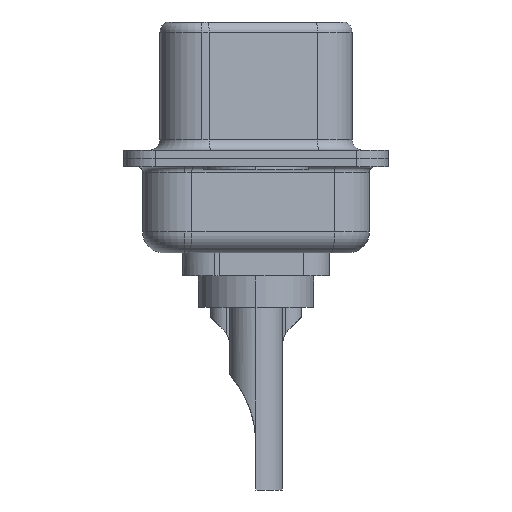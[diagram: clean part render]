
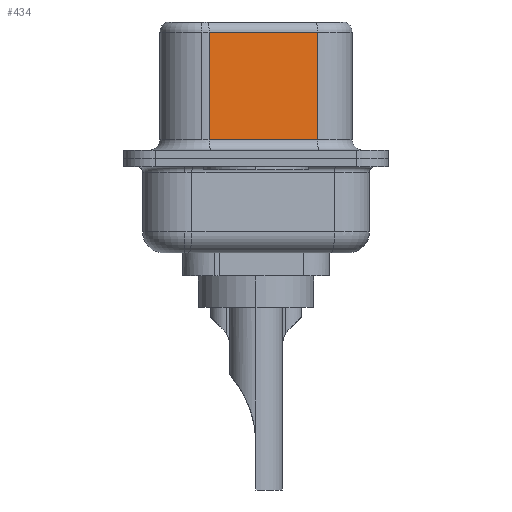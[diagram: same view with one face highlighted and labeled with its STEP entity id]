
A CAD part, left-side view. The second image highlights one B-rep face of the part: STEP entity #434.
In plain terms, the highlighted planar face has unit normal (-0.985, -0.174, 0).
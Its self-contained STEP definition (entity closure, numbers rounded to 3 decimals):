
#17 = DIRECTION ( 'NONE',  ( -0.174, 0.985, 0. ) ) ;
#160 = CARTESIAN_POINT ( 'NONE',  ( 4.565, -2.927, 0.9 ) ) ;
#434 = ADVANCED_FACE ( 'NONE', ( #3321 ), #920, .F. ) ;
#579 = EDGE_CURVE ( 'NONE', #1395, #7417, #12391, .T. ) ;
#673 = LINE ( 'NONE', #160, #12047 ) ;
#817 = DIRECTION ( 'NONE',  ( 0.985, 0.174, 0. ) ) ;
#920 = PLANE ( 'NONE',  #6382 ) ;
#986 = CARTESIAN_POINT ( 'NONE',  ( 4.565, -2.927, 6.02 ) ) ;
#1395 = VERTEX_POINT ( 'NONE', #13186 ) ;
#1412 = CARTESIAN_POINT ( 'NONE',  ( 4.565, -2.927, 6.52 ) ) ;
#2065 = EDGE_CURVE ( 'NONE', #7417, #7648, #2249, .T. ) ;
#2125 = DIRECTION ( 'NONE',  ( -0.174, 0.985, 0. ) ) ;
#2249 = LINE ( 'NONE', #8790, #13193 ) ;
#2367 = DIRECTION ( 'NONE',  ( 0., 0., -1. ) ) ;
#3171 = ORIENTED_EDGE ( 'NONE', *, *, #2065, .T. ) ;
#3321 = FACE_OUTER_BOUND ( 'NONE', #6710, .T. ) ;
#3608 = DIRECTION ( 'NONE',  ( 0., 0., -1. ) ) ;
#3700 = VECTOR ( 'NONE', #2367, 1000. ) ;
#5570 = ORIENTED_EDGE ( 'NONE', *, *, #9872, .F. ) ;
#5875 = CARTESIAN_POINT ( 'NONE',  ( 3.655, 2.233, 6.02 ) ) ;
#6197 = CARTESIAN_POINT ( 'NONE',  ( 3.655, 2.233, 0.9 ) ) ;
#6382 = AXIS2_PLACEMENT_3D ( 'NONE', #1412, #817, #2125 ) ;
#6707 = LINE ( 'NONE', #12182, #3700 ) ;
#6710 = EDGE_LOOP ( 'NONE', ( #5570, #9711, #3171, #8207 ) ) ;
#7417 = VERTEX_POINT ( 'NONE', #5875 ) ;
#7648 = VERTEX_POINT ( 'NONE', #6197 ) ;
#7986 = DIRECTION ( 'NONE',  ( 0.174, -0.985, 0. ) ) ;
#8207 = ORIENTED_EDGE ( 'NONE', *, *, #9887, .T. ) ;
#8790 = CARTESIAN_POINT ( 'NONE',  ( 3.655, 2.233, 6.52 ) ) ;
#9711 = ORIENTED_EDGE ( 'NONE', *, *, #579, .T. ) ;
#9847 = VECTOR ( 'NONE', #17, 1000. ) ;
#9872 = EDGE_CURVE ( 'NONE', #1395, #13435, #6707, .T. ) ;
#9887 = EDGE_CURVE ( 'NONE', #7648, #13435, #673, .T. ) ;
#12047 = VECTOR ( 'NONE', #7986, 1000. ) ;
#12182 = CARTESIAN_POINT ( 'NONE',  ( 4.565, -2.927, 6.52 ) ) ;
#12391 = LINE ( 'NONE', #986, #9847 ) ;
#12587 = CARTESIAN_POINT ( 'NONE',  ( 4.565, -2.927, 0.9 ) ) ;
#13186 = CARTESIAN_POINT ( 'NONE',  ( 4.565, -2.927, 6.02 ) ) ;
#13193 = VECTOR ( 'NONE', #3608, 1000. ) ;
#13435 = VERTEX_POINT ( 'NONE', #12587 ) ;
